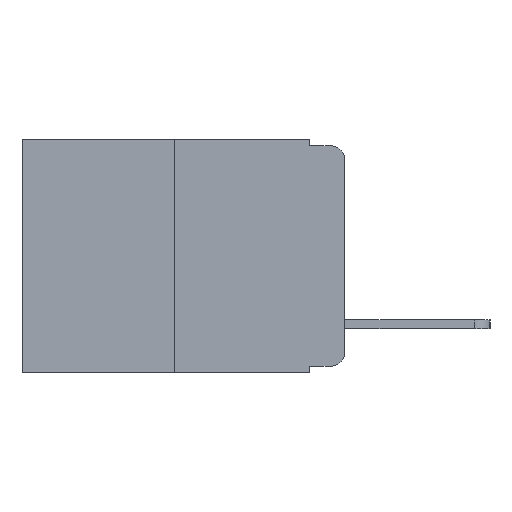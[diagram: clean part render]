
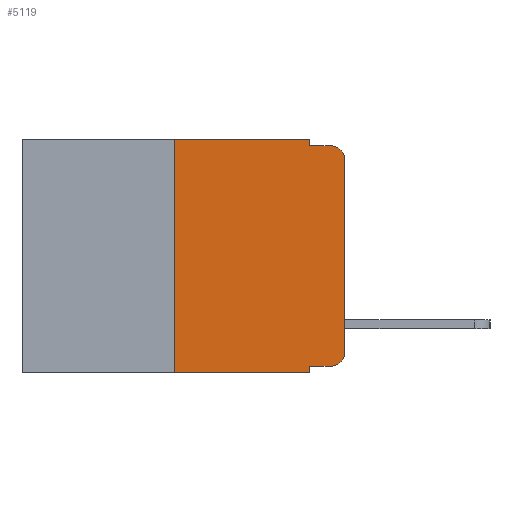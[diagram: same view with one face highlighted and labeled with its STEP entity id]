
A CAD part, left-side view. The second image highlights one B-rep face of the part: STEP entity #5119.
In plain terms, the highlighted planar face has unit normal (-1, 0, 0).
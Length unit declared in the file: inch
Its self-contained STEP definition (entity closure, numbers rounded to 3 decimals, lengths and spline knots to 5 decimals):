
#59 = ORIENTED_EDGE ( 'NONE', *, *, #4455, .T. ) ;
#110 = VERTEX_POINT ( 'NONE', #499 ) ;
#299 = ORIENTED_EDGE ( 'NONE', *, *, #1278, .F. ) ;
#370 = EDGE_CURVE ( 'NONE', #11092, #522, #9095, .T. ) ;
#414 = ORIENTED_EDGE ( 'NONE', *, *, #2668, .F. ) ;
#499 = CARTESIAN_POINT ( 'NONE',  ( 0., 0.051, -0.01 ) ) ;
#522 = VERTEX_POINT ( 'NONE', #10483 ) ;
#696 = CIRCLE ( 'NONE', #961, 0.02 ) ;
#752 = ORIENTED_EDGE ( 'NONE', *, *, #7590, .F. ) ;
#817 = CARTESIAN_POINT ( 'NONE',  ( 0., 0.051, 0. ) ) ;
#835 = CARTESIAN_POINT ( 'NONE',  ( 0., 0.25, 0. ) ) ;
#864 = ORIENTED_EDGE ( 'NONE', *, *, #6907, .F. ) ;
#896 = DIRECTION ( 'NONE',  ( 0., -1., 0. ) ) ;
#932 = ORIENTED_EDGE ( 'NONE', *, *, #2453, .T. ) ;
#961 = AXIS2_PLACEMENT_3D ( 'NONE', #2687, #8755, #3768 ) ;
#1068 = CIRCLE ( 'NONE', #10171, 0.02 ) ;
#1084 = ORIENTED_EDGE ( 'NONE', *, *, #3851, .F. ) ;
#1168 = ORIENTED_EDGE ( 'NONE', *, *, #370, .T. ) ;
#1278 = EDGE_CURVE ( 'NONE', #110, #5989, #9198, .T. ) ;
#1332 = ORIENTED_EDGE ( 'NONE', *, *, #9680, .T. ) ;
#1601 = VERTEX_POINT ( 'NONE', #8990 ) ;
#1615 = VERTEX_POINT ( 'NONE', #8422 ) ;
#1617 = VECTOR ( 'NONE', #5398, 39.37008 ) ;
#1673 = DIRECTION ( 'NONE',  ( 0., 0., -1. ) ) ;
#1960 = DIRECTION ( 'NONE',  ( 0., 0., 1. ) ) ;
#2173 = VECTOR ( 'NONE', #9674, 39.37008 ) ;
#2186 = DIRECTION ( 'NONE',  ( 0., 0., 1. ) ) ;
#2198 = PLANE ( 'NONE',  #7423 ) ;
#2231 = VECTOR ( 'NONE', #5714, 39.37008 ) ;
#2414 = VERTEX_POINT ( 'NONE', #835 ) ;
#2453 = EDGE_CURVE ( 'NONE', #10142, #1601, #4354, .T. ) ;
#2504 = ORIENTED_EDGE ( 'NONE', *, *, #6720, .T. ) ;
#2668 = EDGE_CURVE ( 'NONE', #3803, #110, #6231, .T. ) ;
#2687 = CARTESIAN_POINT ( 'NONE',  ( 0., 0.02, -0.313 ) ) ;
#3139 = CARTESIAN_POINT ( 'NONE',  ( 0., 0.473, 0. ) ) ;
#3257 = CARTESIAN_POINT ( 'NONE',  ( 0., 0.25, 0. ) ) ;
#3456 = DIRECTION ( 'NONE',  ( 1., 0., 0. ) ) ;
#3659 = VERTEX_POINT ( 'NONE', #8980 ) ;
#3768 = DIRECTION ( 'NONE',  ( 0., 0., -1. ) ) ;
#3803 = VERTEX_POINT ( 'NONE', #817 ) ;
#3851 = EDGE_CURVE ( 'NONE', #11092, #1601, #7057, .T. ) ;
#3902 = VECTOR ( 'NONE', #11022, 39.37008 ) ;
#4056 = LINE ( 'NONE', #3257, #6109 ) ;
#4214 = LINE ( 'NONE', #6594, #9626 ) ;
#4354 = LINE ( 'NONE', #6592, #1617 ) ;
#4455 = EDGE_CURVE ( 'NONE', #3659, #5989, #1068, .T. ) ;
#4921 = CARTESIAN_POINT ( 'NONE',  ( 0., 0.051, -0.01 ) ) ;
#5014 = LINE ( 'NONE', #8943, #6717 ) ;
#5119 = ADVANCED_FACE ( 'NONE', ( #10276 ), #2198, .F. ) ;
#5398 = DIRECTION ( 'NONE',  ( 0., -1., 0. ) ) ;
#5714 = DIRECTION ( 'NONE',  ( 0., 0., -1. ) ) ;
#5960 = CARTESIAN_POINT ( 'NONE',  ( 0., 0.051, 0. ) ) ;
#5989 = VERTEX_POINT ( 'NONE', #7255 ) ;
#6109 = VECTOR ( 'NONE', #2186, 39.37008 ) ;
#6231 = LINE ( 'NONE', #10062, #3902 ) ;
#6592 = CARTESIAN_POINT ( 'NONE',  ( 0., 0.473, -0.343 ) ) ;
#6594 = CARTESIAN_POINT ( 'NONE',  ( 0., 0., 0. ) ) ;
#6717 = VECTOR ( 'NONE', #896, 39.37008 ) ;
#6720 = EDGE_CURVE ( 'NONE', #1615, #3659, #4214, .T. ) ;
#6907 = EDGE_CURVE ( 'NONE', #10142, #2414, #4056, .T. ) ;
#7057 = LINE ( 'NONE', #5960, #2231 ) ;
#7255 = CARTESIAN_POINT ( 'NONE',  ( 0., 0.02, -0.01 ) ) ;
#7423 = AXIS2_PLACEMENT_3D ( 'NONE', #3139, #3456, #1673 ) ;
#7590 = EDGE_CURVE ( 'NONE', #2414, #3803, #5014, .T. ) ;
#8422 = CARTESIAN_POINT ( 'NONE',  ( 0., 0., -0.313 ) ) ;
#8755 = DIRECTION ( 'NONE',  ( -1., 0., 0. ) ) ;
#8819 = DIRECTION ( 'NONE',  ( 0., -1., 0. ) ) ;
#8943 = CARTESIAN_POINT ( 'NONE',  ( 0., 0.473, 0. ) ) ;
#8980 = CARTESIAN_POINT ( 'NONE',  ( 0., 0., -0.03 ) ) ;
#8990 = CARTESIAN_POINT ( 'NONE',  ( 0., 0.051, -0.343 ) ) ;
#9095 = LINE ( 'NONE', #10106, #2173 ) ;
#9198 = LINE ( 'NONE', #4921, #10746 ) ;
#9213 = DIRECTION ( 'NONE',  ( 0., 0., -1. ) ) ;
#9239 = DIRECTION ( 'NONE',  ( -1., 0., 0. ) ) ;
#9407 = CARTESIAN_POINT ( 'NONE',  ( 0., 0.02, -0.03 ) ) ;
#9626 = VECTOR ( 'NONE', #1960, 39.37008 ) ;
#9674 = DIRECTION ( 'NONE',  ( 0., -1., 0. ) ) ;
#9680 = EDGE_CURVE ( 'NONE', #522, #1615, #696, .T. ) ;
#9876 = CARTESIAN_POINT ( 'NONE',  ( 0., 0.25, -0.343 ) ) ;
#10062 = CARTESIAN_POINT ( 'NONE',  ( 0., 0.051, 0. ) ) ;
#10106 = CARTESIAN_POINT ( 'NONE',  ( 0., 0.051, -0.333 ) ) ;
#10107 = EDGE_LOOP ( 'NONE', ( #2504, #59, #299, #414, #752, #864, #932, #1084, #1168, #1332 ) ) ;
#10142 = VERTEX_POINT ( 'NONE', #9876 ) ;
#10171 = AXIS2_PLACEMENT_3D ( 'NONE', #9407, #9239, #9213 ) ;
#10276 = FACE_OUTER_BOUND ( 'NONE', #10107, .T. ) ;
#10310 = CARTESIAN_POINT ( 'NONE',  ( 0., 0.051, -0.333 ) ) ;
#10483 = CARTESIAN_POINT ( 'NONE',  ( 0., 0.02, -0.333 ) ) ;
#10746 = VECTOR ( 'NONE', #8819, 39.37008 ) ;
#11022 = DIRECTION ( 'NONE',  ( 0., 0., -1. ) ) ;
#11092 = VERTEX_POINT ( 'NONE', #10310 ) ;
